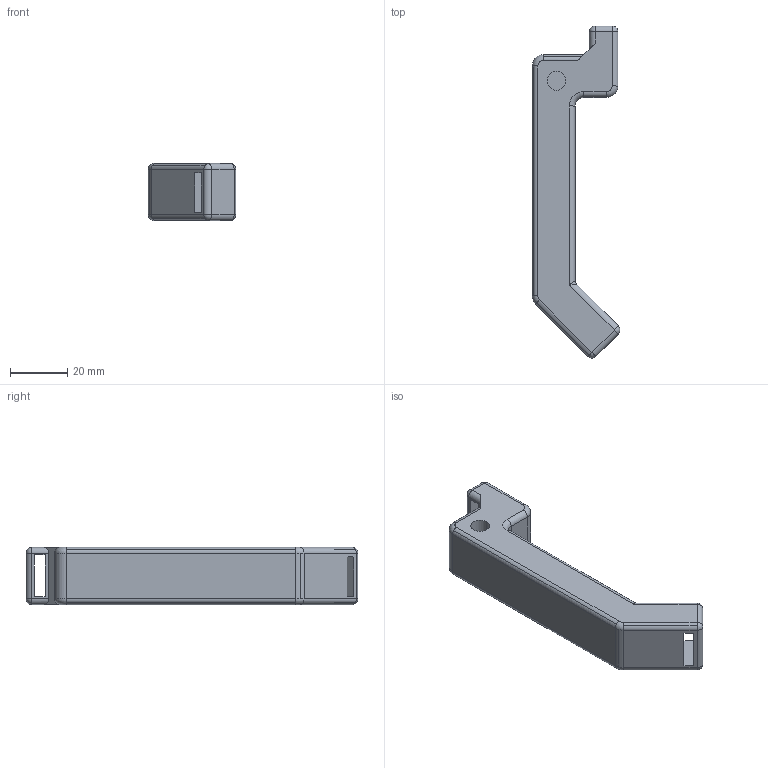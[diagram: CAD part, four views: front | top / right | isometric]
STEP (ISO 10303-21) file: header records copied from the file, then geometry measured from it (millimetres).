
FILE_DESCRIPTION(('STEP AP214'),'1');
FILE_NAME('PBW Brace V0.4 Angled.stp','2020-07-11T02:08:02',(' '),(' '),'Spatial InterOp 3D',' ',' ');
FILE_SCHEMA(('AUTOMOTIVE_DESIGN { 1 0 10303 214 1 1 1 1 }'));
Length unit declared in the file: metre
Products named in the file (1): Body
Bounding box: 30.66 x 116.16 x 20 mm (x, y, z)
Volume: 37003.7 mm3; surface area: 10164.5 mm2
Topology: 1 solids, 1 shells, 79 faces, 192 edges, 106 vertices
Faces by surface type: cylinder 39, plane 22, torus 8, sphere 8, bspline 2
Entity records: 2687 total; most frequent: CARTESIAN_POINT 814, DIRECTION 424, ORIENTED_EDGE 364, EDGE_CURVE 182, AXIS2_PLACEMENT_3D 164, VERTEX_POINT 106, LINE 96, VECTOR 96
